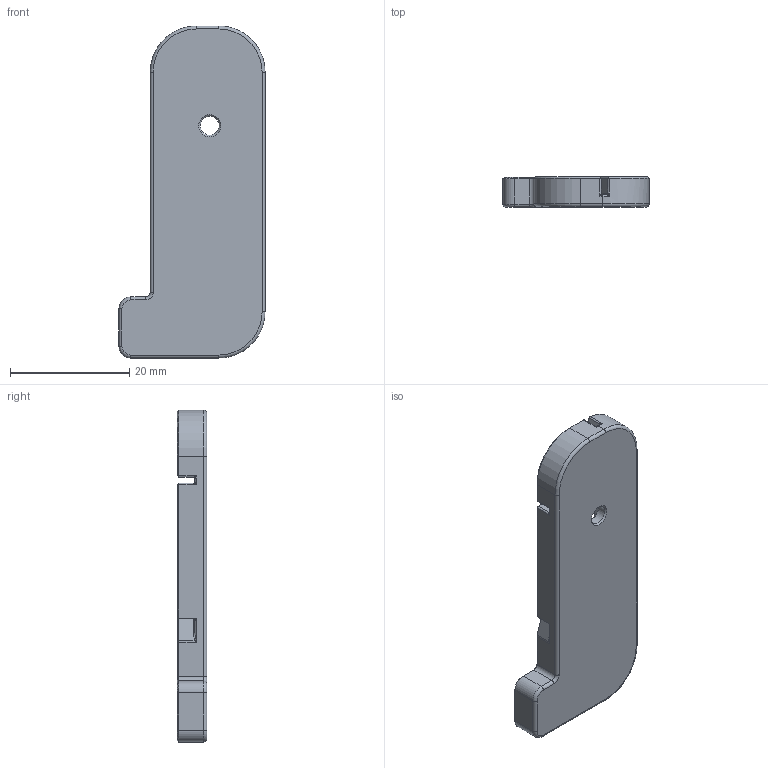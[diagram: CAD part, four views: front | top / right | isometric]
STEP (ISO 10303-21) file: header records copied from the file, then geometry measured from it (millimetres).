
FILE_DESCRIPTION(/* description */ (''),/* implementation_level */ '2;1');
FILE_NAME(/* name */ '2cab06c4-abc2-48a5-8783-03b9be2983c6.stp',/* time_stamp */ '2019-04-26T13:11:20-04:00',/* author */ ('suzuki450ltr'),/* organization */ (''),/* preprocessor_version */ 'ST-DEVELOPER v18',/* originating_system */ 'Autodesk Translation Framework v8.2.0.1029',/* authorisation */ '');
FILE_SCHEMA (('AUTOMOTIVE_DESIGN { 1 0 10303 214 3 1 1 }'));
Length unit declared in the file: millimetre
Products named in the file (1): Ejector Moddification Jig
Bounding box: 24.55 x 5 x 55.75 mm (x, y, z)
Volume: 4188 mm3; surface area: 3437.5 mm2
Topology: 1 solids, 1 shells, 212 faces, 491 edges, 259 vertices
Faces by surface type: cylinder 70, plane 70, cone 35, torus 26, bspline 11
Full cylindrical faces by diameter (mm): 3.175 x1, 5.8 x1
Entity records: 5978 total; most frequent: CARTESIAN_POINT 1269, DIRECTION 1046, ORIENTED_EDGE 932, EDGE_CURVE 466, AXIS2_PLACEMENT_3D 390, LINE 266, VECTOR 266, VERTEX_POINT 259
